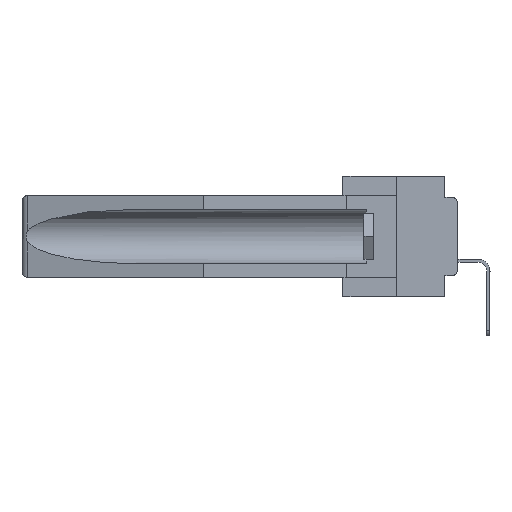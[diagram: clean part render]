
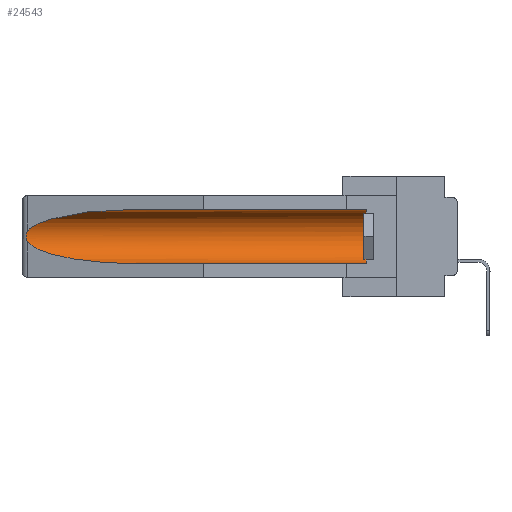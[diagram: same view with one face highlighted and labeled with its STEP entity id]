
A CAD part, left-side view. The second image highlights one B-rep face of the part: STEP entity #24543.
In plain terms, the highlighted cylindrical face has radius 2.857 mm (diameter 5.715 mm), a partial arc.
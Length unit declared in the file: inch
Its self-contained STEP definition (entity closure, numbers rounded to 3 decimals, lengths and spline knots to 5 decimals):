
#82 = ORIENTED_EDGE ( 'NONE', *, *, #35121, .T. ) ;
#545 = CARTESIAN_POINT ( 'NONE',  ( 0.26537, 1.52718, -0.19328 ) ) ;
#604 = CARTESIAN_POINT ( 'NONE',  ( 0.155, -0.30754, -0.059 ) ) ;
#670 = CARTESIAN_POINT ( 'NONE',  ( 0.25451, 1.48313, -0.24835 ) ) ;
#765 = LINE ( 'NONE', #13616, #17773 ) ;
#1046 = CARTESIAN_POINT ( 'NONE',  ( 0.25451, 1.48313, -0.09465 ) ) ;
#1606 = CARTESIAN_POINT ( 'NONE',  ( 0.26655, 1.53094, -0.18657 ) ) ;
#1769 = EDGE_CURVE ( 'NONE', #11748, #19564, #765, .T. ) ;
#1876 = DIRECTION ( 'NONE',  ( 0., 1., 0. ) ) ;
#2051 = EDGE_CURVE ( 'NONE', #24871, #20738, #2958, .T. ) ;
#2816 = EDGE_CURVE ( 'NONE', #20738, #33585, #24292, .T. ) ;
#2866 = CARTESIAN_POINT ( 'NONE',  ( 0.26537, 1.52718, -0.19328 ) ) ;
#2958 = LINE ( 'NONE', #604, #21775 ) ;
#3118 = AXIS2_PLACEMENT_3D ( 'NONE', #36499, #10729, #22112 ) ;
#6982 = EDGE_LOOP ( 'NONE', ( #13003, #82, #25164, #10038, #29385, #32519 ) ) ;
#7612 = CARTESIAN_POINT ( 'NONE',  ( 0.26537, 1.52718, -0.19328 ) ) ;
#8201 = B_SPLINE_CURVE_WITH_KNOTS ( 'NONE', 3,
 ( #18512, #26921, #12634, #24281, #27173, #24415, #18767, #1606, #16116, #7612 ),
 .UNSPECIFIED., .F., .F.,
 ( 4, 2, 2, 2, 4 ),
 ( 0., 0.00029, 0.00058, 0.00087, 0.00117 ),
 .UNSPECIFIED. ) ;
#10030 = CARTESIAN_POINT ( 'NONE',  ( 0.26537, 1.52718, -0.14972 ) ) ;
#10038 = ORIENTED_EDGE ( 'NONE', *, *, #1769, .F. ) ;
#10525 = CARTESIAN_POINT ( 'NONE',  ( 0.155, -0.30754, -0.1715 ) ) ;
#10687 = VERTEX_POINT ( 'NONE', #2866 ) ;
#10729 = DIRECTION ( 'NONE',  ( 0., -1., 0. ) ) ;
#11748 = VERTEX_POINT ( 'NONE', #29172 ) ;
#12560 = CARTESIAN_POINT ( 'NONE',  ( 0.21114, 1.30732, -0.059 ) ) ;
#12634 = CARTESIAN_POINT ( 'NONE',  ( 0.26654, 1.53092, -0.15636 ) ) ;
#12801 = CARTESIAN_POINT ( 'NONE',  ( 0.155, 1.07973, -0.059 ) ) ;
#13003 = ORIENTED_EDGE ( 'NONE', *, *, #2816, .T. ) ;
#13238 = CARTESIAN_POINT ( 'NONE',  ( 0.155, 1.07973, -0.059 ) ) ;
#13616 = CARTESIAN_POINT ( 'NONE',  ( 0.155, -0.30754, -0.284 ) ) ;
#16116 = CARTESIAN_POINT ( 'NONE',  ( 0.26597, 1.5296, -0.19026 ) ) ;
#16605 = CARTESIAN_POINT ( 'NONE',  ( 0.26537, 1.52718, -0.14972 ) ) ;
#17773 = VECTOR ( 'NONE', #19258, 39.37008 ) ;
#18391 = CARTESIAN_POINT ( 'NONE',  ( 0.155, 0.126, -0.059 ) ) ;
#18512 = CARTESIAN_POINT ( 'NONE',  ( 0.26537, 1.52718, -0.14972 ) ) ;
#18767 = CARTESIAN_POINT ( 'NONE',  ( 0.2673, 1.53269, -0.17917 ) ) ;
#19258 = DIRECTION ( 'NONE',  ( 0., 1., 0. ) ) ;
#19564 = VERTEX_POINT ( 'NONE', #26780 ) ;
#20372 =( BOUNDED_CURVE ( )  B_SPLINE_CURVE ( 3, ( #545, #670, #32203, #34944 ),
 .UNSPECIFIED., .F., .F. ) 
 B_SPLINE_CURVE_WITH_KNOTS ( ( 4, 4 ),
 ( 0.1948, 1.5708 ),
 .UNSPECIFIED. ) 
 CURVE ( )  GEOMETRIC_REPRESENTATION_ITEM ( )  RATIONAL_B_SPLINE_CURVE ( ( 1., 0.848, 0.848, 1. ) ) 
 REPRESENTATION_ITEM ( '' )  );
#20738 = VERTEX_POINT ( 'NONE', #13238 ) ;
#21775 = VECTOR ( 'NONE', #23386, 39.37008 ) ;
#21925 = DIRECTION ( 'NONE',  ( 0., 0., 1. ) ) ;
#21984 = AXIS2_PLACEMENT_3D ( 'NONE', #10525, #1876, #21925 ) ;
#22112 = DIRECTION ( 'NONE',  ( 0., 0., 1. ) ) ;
#23386 = DIRECTION ( 'NONE',  ( 0., 1., 0. ) ) ;
#24281 = CARTESIAN_POINT ( 'NONE',  ( 0.2673, 1.5327, -0.16383 ) ) ;
#24292 =( BOUNDED_CURVE ( )  B_SPLINE_CURVE ( 3, ( #12801, #12560, #1046, #10030 ),
 .UNSPECIFIED., .F., .T. ) 
 B_SPLINE_CURVE_WITH_KNOTS ( ( 4, 4 ),
 ( 4.71239, 6.08839 ),
 .UNSPECIFIED. ) 
 CURVE ( )  GEOMETRIC_REPRESENTATION_ITEM ( )  RATIONAL_B_SPLINE_CURVE ( ( 1., 0.848, 0.848, 1. ) ) 
 REPRESENTATION_ITEM ( '' )  );
#24399 = FACE_OUTER_BOUND ( 'NONE', #6982, .T. ) ;
#24415 = CARTESIAN_POINT ( 'NONE',  ( 0.2675, 1.53308, -0.17534 ) ) ;
#24543 = ADVANCED_FACE ( 'NONE', ( #24399 ), #26619, .F. ) ;
#24871 = VERTEX_POINT ( 'NONE', #18391 ) ;
#25164 = ORIENTED_EDGE ( 'NONE', *, *, #26015, .T. ) ;
#26015 = EDGE_CURVE ( 'NONE', #10687, #19564, #20372, .T. ) ;
#26619 = CYLINDRICAL_SURFACE ( 'NONE', #21984, 0.1125 ) ;
#26780 = CARTESIAN_POINT ( 'NONE',  ( 0.155, 1.07973, -0.284 ) ) ;
#26921 = CARTESIAN_POINT ( 'NONE',  ( 0.26597, 1.52961, -0.15275 ) ) ;
#27173 = CARTESIAN_POINT ( 'NONE',  ( 0.2675, 1.53308, -0.16763 ) ) ;
#28717 = EDGE_CURVE ( 'NONE', #11748, #24871, #34724, .T. ) ;
#29172 = CARTESIAN_POINT ( 'NONE',  ( 0.155, 0.126, -0.284 ) ) ;
#29385 = ORIENTED_EDGE ( 'NONE', *, *, #28717, .T. ) ;
#32203 = CARTESIAN_POINT ( 'NONE',  ( 0.21114, 1.30732, -0.284 ) ) ;
#32519 = ORIENTED_EDGE ( 'NONE', *, *, #2051, .T. ) ;
#33585 = VERTEX_POINT ( 'NONE', #16605 ) ;
#34724 = CIRCLE ( 'NONE', #3118, 0.1125 ) ;
#34944 = CARTESIAN_POINT ( 'NONE',  ( 0.155, 1.07973, -0.284 ) ) ;
#35121 = EDGE_CURVE ( 'NONE', #33585, #10687, #8201, .T. ) ;
#36499 = CARTESIAN_POINT ( 'NONE',  ( 0.155, 0.126, -0.1715 ) ) ;
